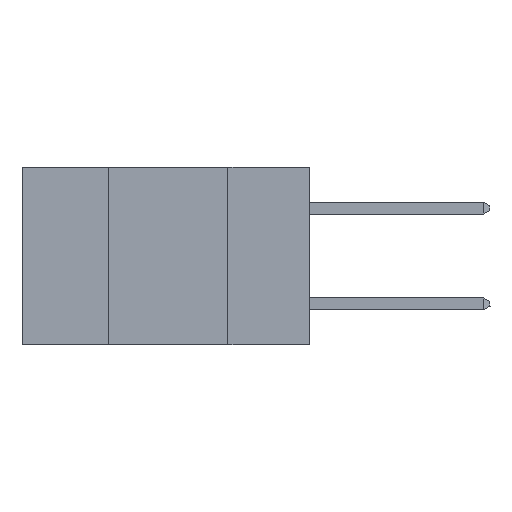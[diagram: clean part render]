
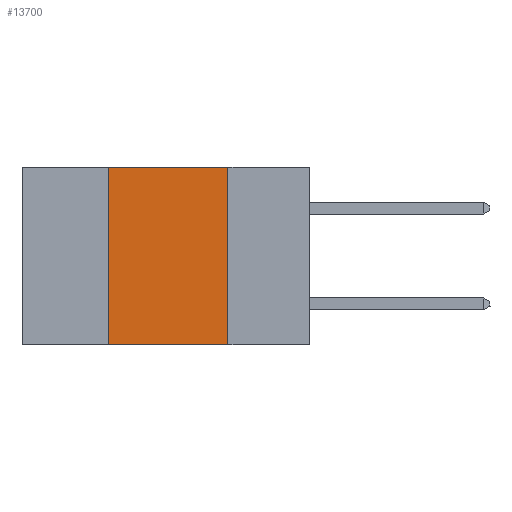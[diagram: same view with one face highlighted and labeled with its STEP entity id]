
A CAD part, left-side view. The second image highlights one B-rep face of the part: STEP entity #13700.
In plain terms, the highlighted planar face has unit normal (-1, 0, 0).
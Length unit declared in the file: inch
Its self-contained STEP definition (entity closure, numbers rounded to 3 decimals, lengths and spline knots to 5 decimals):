
#1581 = CARTESIAN_POINT ( 'NONE',  ( 0., 0.17, 0. ) ) ;
#1671 = ORIENTED_EDGE ( 'NONE', *, *, #9953, .T. ) ;
#2031 = CARTESIAN_POINT ( 'NONE',  ( 0., 0.6, -0.37 ) ) ;
#2315 = ORIENTED_EDGE ( 'NONE', *, *, #14675, .F. ) ;
#2457 = FACE_OUTER_BOUND ( 'NONE', #6918, .T. ) ;
#3589 = DIRECTION ( 'NONE',  ( 0., -1., 0. ) ) ;
#4176 = ORIENTED_EDGE ( 'NONE', *, *, #6153, .F. ) ;
#5494 = LINE ( 'NONE', #1581, #14608 ) ;
#5567 = ORIENTED_EDGE ( 'NONE', *, *, #12380, .F. ) ;
#5994 = CARTESIAN_POINT ( 'NONE',  ( 0., 0.17, -0.37 ) ) ;
#6011 = VERTEX_POINT ( 'NONE', #5994 ) ;
#6153 = EDGE_CURVE ( 'NONE', #7568, #6011, #5494, .T. ) ;
#6302 = CARTESIAN_POINT ( 'NONE',  ( 0., 0.6, 0. ) ) ;
#6389 = LINE ( 'NONE', #6302, #15711 ) ;
#6639 = PLANE ( 'NONE',  #6738 ) ;
#6738 = AXIS2_PLACEMENT_3D ( 'NONE', #15989, #12190, #17708 ) ;
#6918 = EDGE_LOOP ( 'NONE', ( #4176, #2315, #5567, #1671 ) ) ;
#7568 = VERTEX_POINT ( 'NONE', #17877 ) ;
#7653 = CARTESIAN_POINT ( 'NONE',  ( 0., 0.42, 0. ) ) ;
#7810 = VECTOR ( 'NONE', #13125, 39.37008 ) ;
#9953 = EDGE_CURVE ( 'NONE', #10106, #6011, #14387, .T. ) ;
#10106 = VERTEX_POINT ( 'NONE', #14403 ) ;
#10370 = LINE ( 'NONE', #7653, #13111 ) ;
#10728 = DIRECTION ( 'NONE',  ( 0., 0., 1. ) ) ;
#12190 = DIRECTION ( 'NONE',  ( 1., 0., 0. ) ) ;
#12364 = CARTESIAN_POINT ( 'NONE',  ( 0., 0.42, 0. ) ) ;
#12380 = EDGE_CURVE ( 'NONE', #10106, #15117, #10370, .T. ) ;
#13111 = VECTOR ( 'NONE', #10728, 39.37008 ) ;
#13125 = DIRECTION ( 'NONE',  ( 0., -1., 0. ) ) ;
#13700 = ADVANCED_FACE ( 'NONE', ( #2457 ), #6639, .F. ) ;
#14387 = LINE ( 'NONE', #2031, #7810 ) ;
#14403 = CARTESIAN_POINT ( 'NONE',  ( 0., 0.42, -0.37 ) ) ;
#14608 = VECTOR ( 'NONE', #15296, 39.37008 ) ;
#14675 = EDGE_CURVE ( 'NONE', #15117, #7568, #6389, .T. ) ;
#15117 = VERTEX_POINT ( 'NONE', #12364 ) ;
#15296 = DIRECTION ( 'NONE',  ( 0., 0., -1. ) ) ;
#15711 = VECTOR ( 'NONE', #3589, 39.37008 ) ;
#15989 = CARTESIAN_POINT ( 'NONE',  ( 0., 0.6, 0. ) ) ;
#17708 = DIRECTION ( 'NONE',  ( 0., 0., -1. ) ) ;
#17877 = CARTESIAN_POINT ( 'NONE',  ( 0., 0.17, 0. ) ) ;
